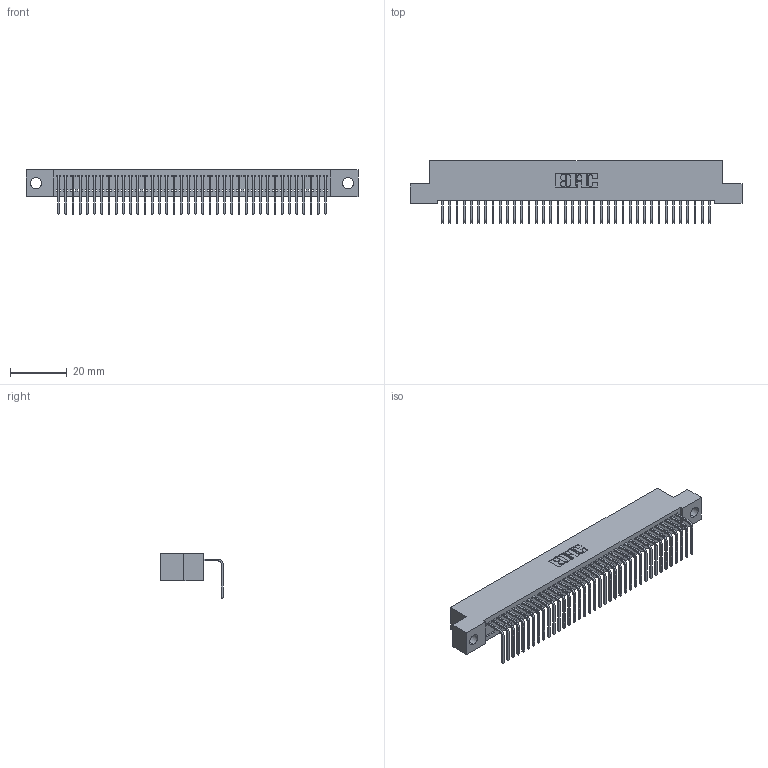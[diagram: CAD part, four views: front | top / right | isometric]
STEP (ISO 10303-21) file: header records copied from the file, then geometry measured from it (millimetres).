
FILE_DESCRIPTION (( 'STEP AP203' ), '1' );
FILE_NAME ('342-038-558-104.STEP', '2019-10-02T15:05:26', ( '' ), ( '' ), 'SwSTEP 2.0', 'SolidWorks 2016', '' );
FILE_SCHEMA (( 'CONFIG_CONTROL_DESIGN' ));
Length unit declared in the file: inch
Products named in the file (3): 342 Part_.156 TH; 345-292-001_558 Tail - 2; 342-038-558-104
Assembly tree (39 placements, depth 2):
  342-038-558-104
    342 Part_.156 TH
    345-292-001_558 Tail - 2  x38
Bounding box: 116.84 x 21.91 x 15.62 mm (x, y, z)
Volume: 10269.4 mm3; surface area: 15543.3 mm2
Topology: 39 solids, 39 shells, 2390 faces, 7215 edges, 4758 vertices
Faces by surface type: plane 1738, cylinder 652
Entity records: 23703 total; most frequent: CARTESIAN_POINT 4096, ORIENTED_EDGE 4070, DIRECTION 3463, EDGE_CURVE 2035, VECTOR 1907, LINE 1907, VERTEX_POINT 1354, AXIS2_PLACEMENT_3D 778
